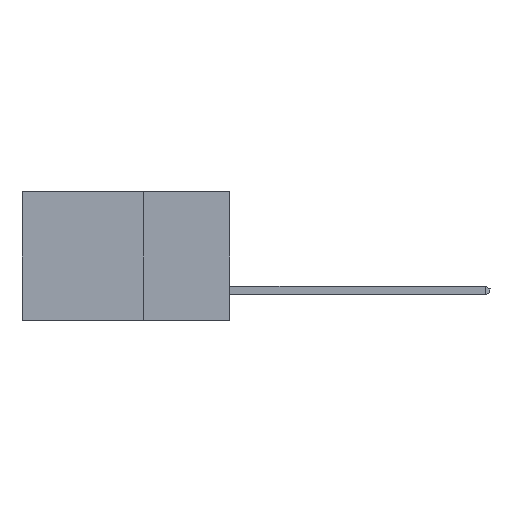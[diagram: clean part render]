
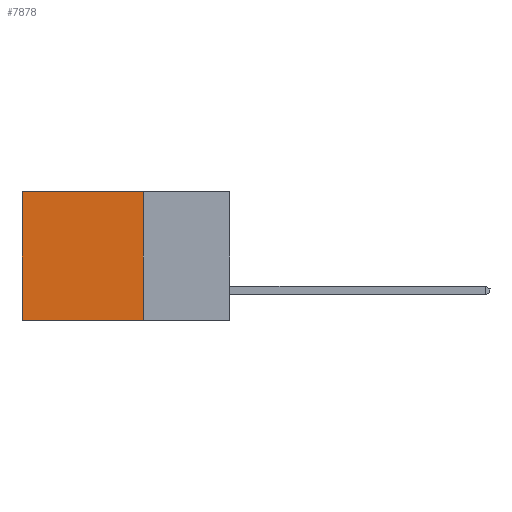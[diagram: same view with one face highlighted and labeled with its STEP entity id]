
A CAD part, left-side view. The second image highlights one B-rep face of the part: STEP entity #7878.
In plain terms, the highlighted planar face has unit normal (-1, 0, 0).
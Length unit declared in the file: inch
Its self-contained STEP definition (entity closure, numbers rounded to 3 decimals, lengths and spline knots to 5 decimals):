
#477 = VERTEX_POINT ( 'NONE', #3534 ) ;
#494 = CARTESIAN_POINT ( 'NONE',  ( 0.2615, 0.25, 0. ) ) ;
#1554 = LINE ( 'NONE', #12783, #19180 ) ;
#1660 = DIRECTION ( 'NONE',  ( 0., 1., 0. ) ) ;
#1771 = CARTESIAN_POINT ( 'NONE',  ( 0.2615, 0.6, -0.37 ) ) ;
#1826 = VECTOR ( 'NONE', #5082, 39.37008 ) ;
#2031 = VERTEX_POINT ( 'NONE', #18497 ) ;
#2646 = DIRECTION ( 'NONE',  ( 0., 0., -1. ) ) ;
#3534 = CARTESIAN_POINT ( 'NONE',  ( 0.2615, 0.25, -0.37 ) ) ;
#3690 = EDGE_CURVE ( 'NONE', #18621, #2031, #7964, .T. ) ;
#4217 = EDGE_LOOP ( 'NONE', ( #10640, #11805, #7726, #13466 ) ) ;
#4473 = CARTESIAN_POINT ( 'NONE',  ( 0.2615, 0.25, -0.37 ) ) ;
#4614 = EDGE_CURVE ( 'NONE', #2031, #18935, #14144, .T. ) ;
#4850 = DIRECTION ( 'NONE',  ( 0., 0., -1. ) ) ;
#5082 = DIRECTION ( 'NONE',  ( 0., 1., 0. ) ) ;
#5281 = EDGE_CURVE ( 'NONE', #18621, #477, #7542, .T. ) ;
#7542 = LINE ( 'NONE', #4473, #13294 ) ;
#7726 = ORIENTED_EDGE ( 'NONE', *, *, #5281, .F. ) ;
#7878 = ADVANCED_FACE ( 'NONE', ( #16389 ), #13583, .F. ) ;
#7964 = LINE ( 'NONE', #494, #1826 ) ;
#9466 = AXIS2_PLACEMENT_3D ( 'NONE', #11557, #10131, #17827 ) ;
#10131 = DIRECTION ( 'NONE',  ( 1., 0., 0. ) ) ;
#10640 = ORIENTED_EDGE ( 'NONE', *, *, #4614, .T. ) ;
#11557 = CARTESIAN_POINT ( 'NONE',  ( 0.2615, 0.25, -0.37 ) ) ;
#11805 = ORIENTED_EDGE ( 'NONE', *, *, #19867, .F. ) ;
#12783 = CARTESIAN_POINT ( 'NONE',  ( 0.2615, 0.25, -0.37 ) ) ;
#13294 = VECTOR ( 'NONE', #2646, 39.37008 ) ;
#13466 = ORIENTED_EDGE ( 'NONE', *, *, #3690, .T. ) ;
#13583 = PLANE ( 'NONE',  #9466 ) ;
#14144 = LINE ( 'NONE', #1771, #14608 ) ;
#14608 = VECTOR ( 'NONE', #4850, 39.37008 ) ;
#15139 = CARTESIAN_POINT ( 'NONE',  ( 0.2615, 0.25, 0. ) ) ;
#16389 = FACE_OUTER_BOUND ( 'NONE', #4217, .T. ) ;
#17827 = DIRECTION ( 'NONE',  ( 0., 0., -1. ) ) ;
#18497 = CARTESIAN_POINT ( 'NONE',  ( 0.2615, 0.6, 0. ) ) ;
#18621 = VERTEX_POINT ( 'NONE', #15139 ) ;
#18935 = VERTEX_POINT ( 'NONE', #19122 ) ;
#19122 = CARTESIAN_POINT ( 'NONE',  ( 0.2615, 0.6, -0.37 ) ) ;
#19180 = VECTOR ( 'NONE', #1660, 39.37008 ) ;
#19867 = EDGE_CURVE ( 'NONE', #477, #18935, #1554, .T. ) ;
